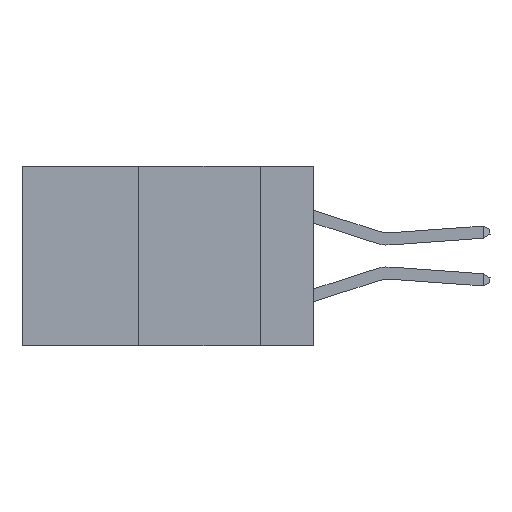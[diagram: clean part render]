
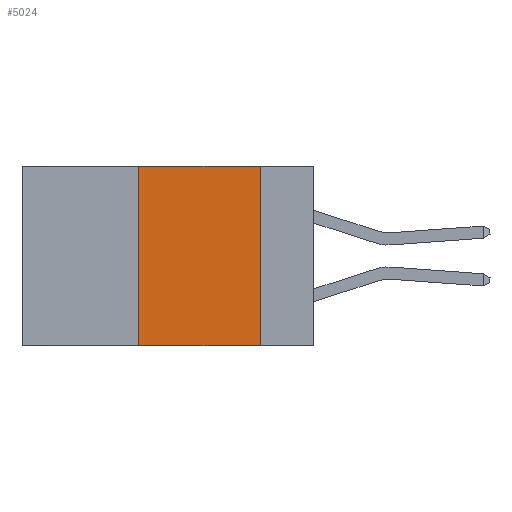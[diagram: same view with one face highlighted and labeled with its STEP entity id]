
A CAD part, left-side view. The second image highlights one B-rep face of the part: STEP entity #5024.
In plain terms, the highlighted planar face has unit normal (-1, 0, 0).
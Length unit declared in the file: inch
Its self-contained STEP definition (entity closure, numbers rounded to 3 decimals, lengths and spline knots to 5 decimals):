
#151 = ORIENTED_EDGE ( 'NONE', *, *, #6176, .F. ) ;
#238 = VECTOR ( 'NONE', #11905, 39.37008 ) ;
#428 = FACE_OUTER_BOUND ( 'NONE', #1595, .T. ) ;
#656 = ORIENTED_EDGE ( 'NONE', *, *, #2721, .F. ) ;
#766 = ORIENTED_EDGE ( 'NONE', *, *, #2075, .T. ) ;
#1381 = CARTESIAN_POINT ( 'NONE',  ( 0., 0.36, 0. ) ) ;
#1595 = EDGE_LOOP ( 'NONE', ( #151, #656, #4673, #766 ) ) ;
#1982 = CARTESIAN_POINT ( 'NONE',  ( 0., 0.36, 0. ) ) ;
#2075 = EDGE_CURVE ( 'NONE', #5562, #13884, #3024, .T. ) ;
#2717 = CARTESIAN_POINT ( 'NONE',  ( 0., 0.6, 0. ) ) ;
#2721 = EDGE_CURVE ( 'NONE', #7701, #8696, #6083, .T. ) ;
#3024 = LINE ( 'NONE', #5165, #6059 ) ;
#3342 = CARTESIAN_POINT ( 'NONE',  ( 0., 0.6, 0. ) ) ;
#4467 = DIRECTION ( 'NONE',  ( 1., 0., 0. ) ) ;
#4673 = ORIENTED_EDGE ( 'NONE', *, *, #12651, .F. ) ;
#5024 = ADVANCED_FACE ( 'NONE', ( #428 ), #11094, .F. ) ;
#5066 = DIRECTION ( 'NONE',  ( 0., -1., 0. ) ) ;
#5165 = CARTESIAN_POINT ( 'NONE',  ( 0., 0.6, -0.37 ) ) ;
#5562 = VERTEX_POINT ( 'NONE', #10857 ) ;
#6059 = VECTOR ( 'NONE', #5066, 39.37008 ) ;
#6083 = LINE ( 'NONE', #2717, #8342 ) ;
#6176 = EDGE_CURVE ( 'NONE', #8696, #13884, #11776, .T. ) ;
#7652 = CARTESIAN_POINT ( 'NONE',  ( 0., 0.11, -0.37 ) ) ;
#7701 = VERTEX_POINT ( 'NONE', #1381 ) ;
#8271 = VECTOR ( 'NONE', #11879, 39.37008 ) ;
#8342 = VECTOR ( 'NONE', #10453, 39.37008 ) ;
#8696 = VERTEX_POINT ( 'NONE', #12638 ) ;
#8728 = CARTESIAN_POINT ( 'NONE',  ( 0., 0.11, 0. ) ) ;
#10453 = DIRECTION ( 'NONE',  ( 0., -1., 0. ) ) ;
#10857 = CARTESIAN_POINT ( 'NONE',  ( 0., 0.36, -0.37 ) ) ;
#11094 = PLANE ( 'NONE',  #11294 ) ;
#11294 = AXIS2_PLACEMENT_3D ( 'NONE', #3342, #4467, #12128 ) ;
#11776 = LINE ( 'NONE', #8728, #8271 ) ;
#11879 = DIRECTION ( 'NONE',  ( 0., 0., -1. ) ) ;
#11905 = DIRECTION ( 'NONE',  ( 0., 0., 1. ) ) ;
#12128 = DIRECTION ( 'NONE',  ( 0., 0., -1. ) ) ;
#12638 = CARTESIAN_POINT ( 'NONE',  ( 0., 0.11, 0. ) ) ;
#12651 = EDGE_CURVE ( 'NONE', #5562, #7701, #14137, .T. ) ;
#13884 = VERTEX_POINT ( 'NONE', #7652 ) ;
#14137 = LINE ( 'NONE', #1982, #238 ) ;
